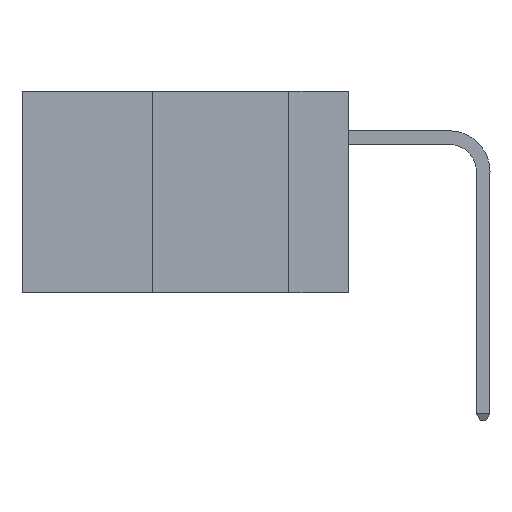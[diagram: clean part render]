
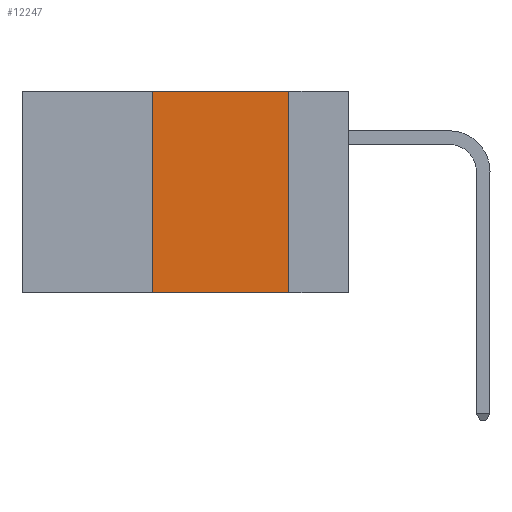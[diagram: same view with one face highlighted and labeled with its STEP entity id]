
A CAD part, left-side view. The second image highlights one B-rep face of the part: STEP entity #12247.
In plain terms, the highlighted planar face has unit normal (-1, 0, 0).
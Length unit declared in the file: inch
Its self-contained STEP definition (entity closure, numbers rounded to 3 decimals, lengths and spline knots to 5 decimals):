
#744 = VECTOR ( 'NONE', #7449, 39.37008 ) ;
#1241 = EDGE_CURVE ( 'NONE', #14351, #21564, #18337, .T. ) ;
#1435 = VERTEX_POINT ( 'NONE', #10033 ) ;
#2242 = DIRECTION ( 'NONE',  ( 0., 0., 1. ) ) ;
#3305 = CARTESIAN_POINT ( 'NONE',  ( 0., 0.6, -0.37 ) ) ;
#4701 = ORIENTED_EDGE ( 'NONE', *, *, #5148, .T. ) ;
#5148 = EDGE_CURVE ( 'NONE', #1435, #25206, #17162, .T. ) ;
#5229 = FACE_OUTER_BOUND ( 'NONE', #27291, .T. ) ;
#6440 = LINE ( 'NONE', #22635, #17044 ) ;
#6561 = VECTOR ( 'NONE', #9897, 39.37008 ) ;
#7449 = DIRECTION ( 'NONE',  ( 0., -1., 0. ) ) ;
#7664 = ORIENTED_EDGE ( 'NONE', *, *, #26780, .F. ) ;
#7706 = PLANE ( 'NONE',  #19874 ) ;
#9823 = CARTESIAN_POINT ( 'NONE',  ( 0., 0.6, 0. ) ) ;
#9897 = DIRECTION ( 'NONE',  ( 0., -1., 0. ) ) ;
#10033 = CARTESIAN_POINT ( 'NONE',  ( 0., 0.36, -0.37 ) ) ;
#11961 = DIRECTION ( 'NONE',  ( 1., 0., 0. ) ) ;
#12062 = DIRECTION ( 'NONE',  ( 0., 0., -1. ) ) ;
#12247 = ADVANCED_FACE ( 'NONE', ( #5229 ), #7706, .F. ) ;
#13003 = ORIENTED_EDGE ( 'NONE', *, *, #13153, .F. ) ;
#13153 = EDGE_CURVE ( 'NONE', #1435, #14351, #25045, .T. ) ;
#14266 = CARTESIAN_POINT ( 'NONE',  ( 0., 0.36, 0. ) ) ;
#14351 = VERTEX_POINT ( 'NONE', #14266 ) ;
#17044 = VECTOR ( 'NONE', #12062, 39.37008 ) ;
#17162 = LINE ( 'NONE', #3305, #6561 ) ;
#17992 = CARTESIAN_POINT ( 'NONE',  ( 0., 0.6, 0. ) ) ;
#18029 = CARTESIAN_POINT ( 'NONE',  ( 0., 0.11, 0. ) ) ;
#18337 = LINE ( 'NONE', #17992, #744 ) ;
#18563 = CARTESIAN_POINT ( 'NONE',  ( 0., 0.11, -0.37 ) ) ;
#19428 = VECTOR ( 'NONE', #2242, 39.37008 ) ;
#19874 = AXIS2_PLACEMENT_3D ( 'NONE', #9823, #11961, #26716 ) ;
#21564 = VERTEX_POINT ( 'NONE', #18029 ) ;
#22635 = CARTESIAN_POINT ( 'NONE',  ( 0., 0.11, 0. ) ) ;
#23391 = CARTESIAN_POINT ( 'NONE',  ( 0., 0.36, 0. ) ) ;
#25045 = LINE ( 'NONE', #23391, #19428 ) ;
#25206 = VERTEX_POINT ( 'NONE', #18563 ) ;
#26716 = DIRECTION ( 'NONE',  ( 0., 0., -1. ) ) ;
#26780 = EDGE_CURVE ( 'NONE', #21564, #25206, #6440, .T. ) ;
#26849 = ORIENTED_EDGE ( 'NONE', *, *, #1241, .F. ) ;
#27291 = EDGE_LOOP ( 'NONE', ( #7664, #26849, #13003, #4701 ) ) ;
